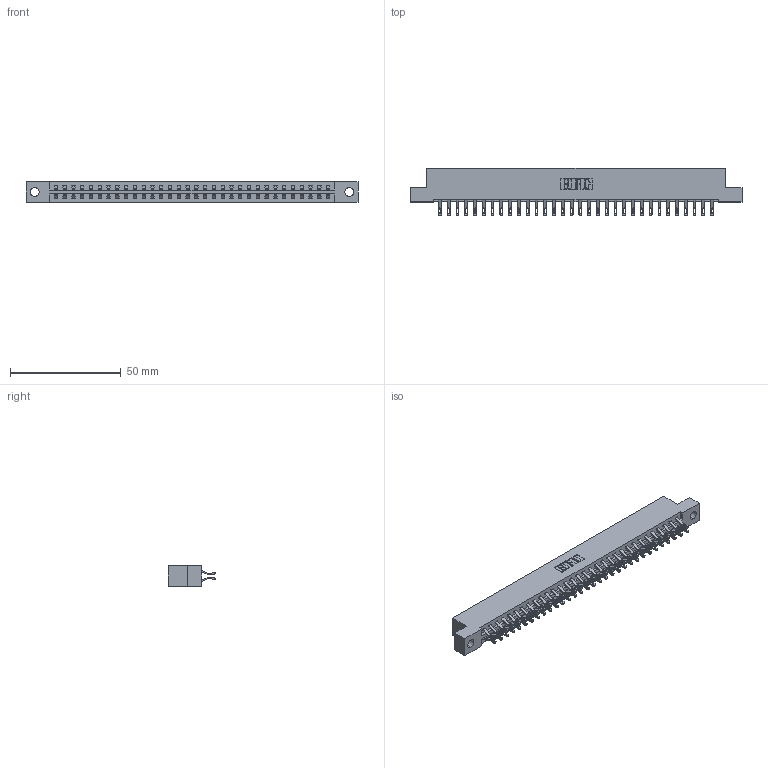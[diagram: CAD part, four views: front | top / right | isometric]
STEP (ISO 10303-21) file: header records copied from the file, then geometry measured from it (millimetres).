
FILE_DESCRIPTION (( 'STEP AP203' ), '1' );
FILE_NAME ('387-064-555-204.STEP', '2018-09-21T08:05:06', ( '' ), ( '' ), 'SwSTEP 2.0', 'SolidWorks 2016', '' );
FILE_SCHEMA (( 'CONFIG_CONTROL_DESIGN' ));
Length unit declared in the file: inch
Products named in the file (3): 337 Part_Flush Mounting Lugs - 0.156 Dia-TH; 345-292-001_555 Tail; 387-064-555-204
Assembly tree (65 placements, depth 2):
  387-064-555-204
    337 Part_Flush Mounting Lugs - 0.156 Dia-TH
    345-292-001_555 Tail  x64
Bounding box: 149.81 x 21.47 x 9.4 mm (x, y, z)
Volume: 15752.7 mm3; surface area: 18208.3 mm2
Topology: 65 solids, 65 shells, 3954 faces, 12407 edges, 8270 vertices
Faces by surface type: plane 2374, cylinder 1580
Entity records: 26433 total; most frequent: CARTESIAN_POINT 4496, ORIENTED_EDGE 4402, DIRECTION 3813, EDGE_CURVE 2201, VECTOR 2053, LINE 2053, VERTEX_POINT 1466, AXIS2_PLACEMENT_3D 880
